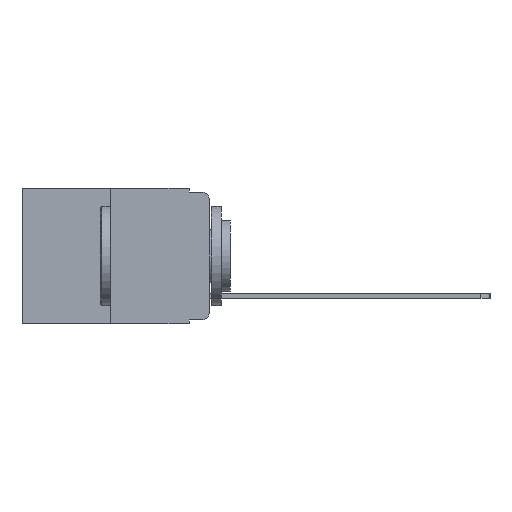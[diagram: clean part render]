
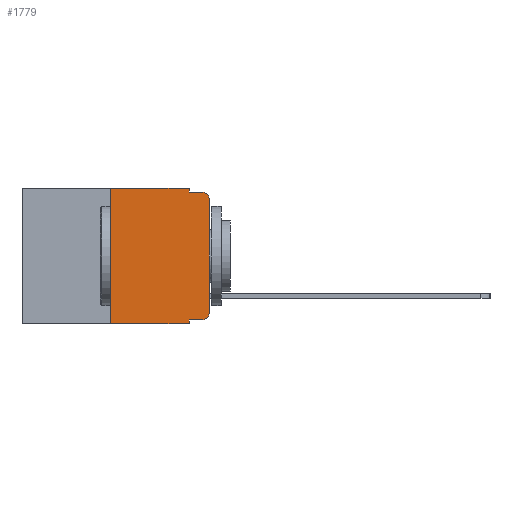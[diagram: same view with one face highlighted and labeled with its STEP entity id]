
A CAD part, left-side view. The second image highlights one B-rep face of the part: STEP entity #1779.
In plain terms, the highlighted planar face has unit normal (-1, 0, 0).
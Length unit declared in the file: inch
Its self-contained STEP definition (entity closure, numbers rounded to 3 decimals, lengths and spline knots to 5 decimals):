
#59 = VERTEX_POINT ( 'NONE', #3078 ) ;
#203 = LINE ( 'NONE', #3879, #4829 ) ;
#306 = CARTESIAN_POINT ( 'NONE',  ( 0., 0.25, -0.343 ) ) ;
#430 = DIRECTION ( 'NONE',  ( 0., -1., 0. ) ) ;
#1306 = DIRECTION ( 'NONE',  ( 0., 0., 1. ) ) ;
#1779 = ADVANCED_FACE ( 'NONE', ( #14492 ), #21658, .F. ) ;
#2271 = VERTEX_POINT ( 'NONE', #4022 ) ;
#2322 = CARTESIAN_POINT ( 'NONE',  ( 0., 0.02, -0.01 ) ) ;
#2806 = ORIENTED_EDGE ( 'NONE', *, *, #18860, .T. ) ;
#2819 = LINE ( 'NONE', #7140, #22766 ) ;
#2839 = LINE ( 'NONE', #12179, #13238 ) ;
#3078 = CARTESIAN_POINT ( 'NONE',  ( 0., 0.25, 0. ) ) ;
#3157 = EDGE_CURVE ( 'NONE', #10932, #2271, #2819, .T. ) ;
#3481 = ORIENTED_EDGE ( 'NONE', *, *, #20379, .T. ) ;
#3527 = CARTESIAN_POINT ( 'NONE',  ( 0., 0.02, -0.333 ) ) ;
#3706 = ORIENTED_EDGE ( 'NONE', *, *, #5927, .T. ) ;
#3763 = CIRCLE ( 'NONE', #6045, 0.02 ) ;
#3879 = CARTESIAN_POINT ( 'NONE',  ( 0., 0., 0. ) ) ;
#4022 = CARTESIAN_POINT ( 'NONE',  ( 0., 0.051, -0.343 ) ) ;
#4211 = VECTOR ( 'NONE', #10576, 39.37008 ) ;
#4588 = EDGE_LOOP ( 'NONE', ( #3706, #2806, #20685, #9597, #18301, #16824, #3481, #17447, #12523, #11049 ) ) ;
#4829 = VECTOR ( 'NONE', #1306, 39.37008 ) ;
#5306 = CARTESIAN_POINT ( 'NONE',  ( 0., 0.473, -0.343 ) ) ;
#5314 = VERTEX_POINT ( 'NONE', #306 ) ;
#5634 = CARTESIAN_POINT ( 'NONE',  ( 0., 0.051, 0. ) ) ;
#5927 = EDGE_CURVE ( 'NONE', #12808, #15036, #203, .T. ) ;
#6045 = AXIS2_PLACEMENT_3D ( 'NONE', #20003, #8479, #21879 ) ;
#6195 = CARTESIAN_POINT ( 'NONE',  ( 0., 0., -0.03 ) ) ;
#6354 = AXIS2_PLACEMENT_3D ( 'NONE', #21451, #6679, #6773 ) ;
#6679 = DIRECTION ( 'NONE',  ( 1., 0., 0. ) ) ;
#6773 = DIRECTION ( 'NONE',  ( 0., 0., -1. ) ) ;
#7105 = DIRECTION ( 'NONE',  ( 0., 0., 1. ) ) ;
#7140 = CARTESIAN_POINT ( 'NONE',  ( 0., 0.051, 0. ) ) ;
#7949 = VECTOR ( 'NONE', #22974, 39.37008 ) ;
#8071 = DIRECTION ( 'NONE',  ( 0., 0., -1. ) ) ;
#8331 = VECTOR ( 'NONE', #7105, 39.37008 ) ;
#8479 = DIRECTION ( 'NONE',  ( -1., 0., 0. ) ) ;
#8612 = CARTESIAN_POINT ( 'NONE',  ( 0., 0., -0.313 ) ) ;
#9028 = AXIS2_PLACEMENT_3D ( 'NONE', #21899, #10457, #23839 ) ;
#9120 = VECTOR ( 'NONE', #10549, 39.37008 ) ;
#9269 = DIRECTION ( 'NONE',  ( 0., -1., 0. ) ) ;
#9287 = EDGE_CURVE ( 'NONE', #17354, #12808, #13965, .T. ) ;
#9592 = CARTESIAN_POINT ( 'NONE',  ( 0., 0.051, -0.333 ) ) ;
#9597 = ORIENTED_EDGE ( 'NONE', *, *, #15808, .F. ) ;
#10457 = DIRECTION ( 'NONE',  ( -1., 0., 0. ) ) ;
#10549 = DIRECTION ( 'NONE',  ( 0., -1., 0. ) ) ;
#10576 = DIRECTION ( 'NONE',  ( 0., 0., -1. ) ) ;
#10739 = VECTOR ( 'NONE', #9269, 39.37008 ) ;
#10932 = VERTEX_POINT ( 'NONE', #23408 ) ;
#11049 = ORIENTED_EDGE ( 'NONE', *, *, #9287, .T. ) ;
#12179 = CARTESIAN_POINT ( 'NONE',  ( 0., 0.051, -0.01 ) ) ;
#12523 = ORIENTED_EDGE ( 'NONE', *, *, #21289, .T. ) ;
#12808 = VERTEX_POINT ( 'NONE', #8612 ) ;
#13238 = VECTOR ( 'NONE', #430, 39.37008 ) ;
#13460 = LINE ( 'NONE', #14782, #8331 ) ;
#13965 = CIRCLE ( 'NONE', #9028, 0.02 ) ;
#14098 = EDGE_CURVE ( 'NONE', #5314, #59, #13460, .T. ) ;
#14492 = FACE_OUTER_BOUND ( 'NONE', #4588, .T. ) ;
#14591 = LINE ( 'NONE', #9592, #7949 ) ;
#14782 = CARTESIAN_POINT ( 'NONE',  ( 0., 0.25, 0. ) ) ;
#15036 = VERTEX_POINT ( 'NONE', #6195 ) ;
#15449 = VERTEX_POINT ( 'NONE', #22803 ) ;
#15808 = EDGE_CURVE ( 'NONE', #24091, #15449, #18454, .T. ) ;
#15826 = LINE ( 'NONE', #5306, #10739 ) ;
#16440 = EDGE_CURVE ( 'NONE', #59, #24091, #18728, .T. ) ;
#16824 = ORIENTED_EDGE ( 'NONE', *, *, #14098, .F. ) ;
#17354 = VERTEX_POINT ( 'NONE', #3527 ) ;
#17447 = ORIENTED_EDGE ( 'NONE', *, *, #3157, .F. ) ;
#17580 = VERTEX_POINT ( 'NONE', #2322 ) ;
#18301 = ORIENTED_EDGE ( 'NONE', *, *, #16440, .F. ) ;
#18454 = LINE ( 'NONE', #22029, #4211 ) ;
#18728 = LINE ( 'NONE', #21998, #9120 ) ;
#18860 = EDGE_CURVE ( 'NONE', #15036, #17580, #3763, .T. ) ;
#20003 = CARTESIAN_POINT ( 'NONE',  ( 0., 0.02, -0.03 ) ) ;
#20379 = EDGE_CURVE ( 'NONE', #5314, #2271, #15826, .T. ) ;
#20685 = ORIENTED_EDGE ( 'NONE', *, *, #23973, .F. ) ;
#21289 = EDGE_CURVE ( 'NONE', #10932, #17354, #14591, .T. ) ;
#21451 = CARTESIAN_POINT ( 'NONE',  ( 0., 0.473, 0. ) ) ;
#21658 = PLANE ( 'NONE',  #6354 ) ;
#21879 = DIRECTION ( 'NONE',  ( 0., 0., -1. ) ) ;
#21899 = CARTESIAN_POINT ( 'NONE',  ( 0., 0.02, -0.313 ) ) ;
#21998 = CARTESIAN_POINT ( 'NONE',  ( 0., 0.473, 0. ) ) ;
#22029 = CARTESIAN_POINT ( 'NONE',  ( 0., 0.051, 0. ) ) ;
#22766 = VECTOR ( 'NONE', #8071, 39.37008 ) ;
#22803 = CARTESIAN_POINT ( 'NONE',  ( 0., 0.051, -0.01 ) ) ;
#22974 = DIRECTION ( 'NONE',  ( 0., -1., 0. ) ) ;
#23408 = CARTESIAN_POINT ( 'NONE',  ( 0., 0.051, -0.333 ) ) ;
#23839 = DIRECTION ( 'NONE',  ( 0., 0., -1. ) ) ;
#23973 = EDGE_CURVE ( 'NONE', #15449, #17580, #2839, .T. ) ;
#24091 = VERTEX_POINT ( 'NONE', #5634 ) ;
